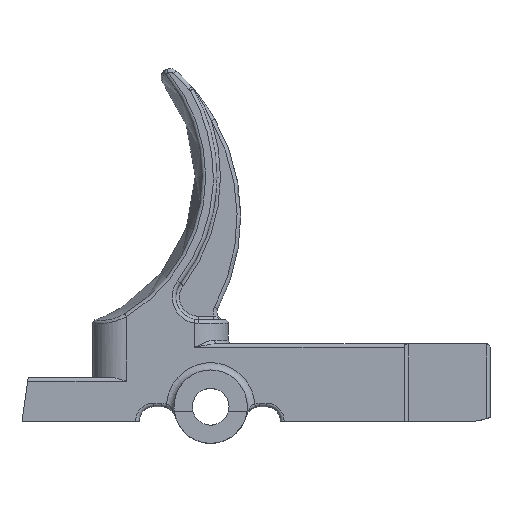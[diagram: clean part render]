
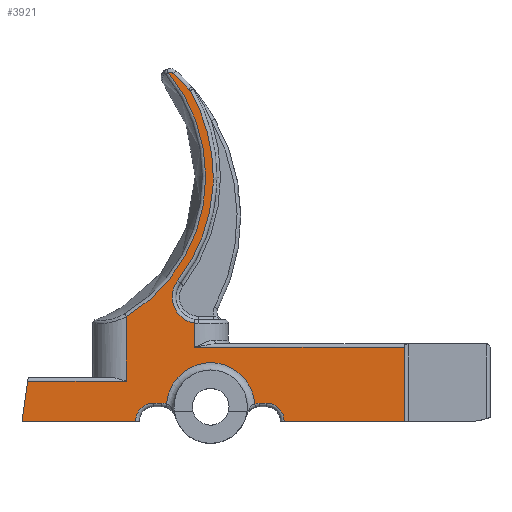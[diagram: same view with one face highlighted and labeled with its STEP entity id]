
A CAD part, top view. The second image highlights one B-rep face of the part: STEP entity #3921.
In plain terms, the highlighted planar face has unit normal (0, 0, 1).
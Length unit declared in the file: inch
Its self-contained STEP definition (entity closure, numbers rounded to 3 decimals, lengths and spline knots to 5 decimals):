
#43=DIRECTION('',(-1.,0.,0.));
#44=VECTOR('',#43,0.5164);
#45=CARTESIAN_POINT('',(1.19332,-0.3337,0.145));
#46=LINE('',#45,#44);
#96=CARTESIAN_POINT('',(0.59932,-0.332,0.145));
#97=DIRECTION('',(0.,0.,-1.));
#98=DIRECTION('',(0.,1.,0.));
#99=AXIS2_PLACEMENT_3D('',#96,#97,#98);
#104=CARTESIAN_POINT('',(0.57196,-0.332,0.145));
#105=DIRECTION('',(0.,0.,-1.));
#106=DIRECTION('',(-0.277,0.961,0.));
#107=AXIS2_PLACEMENT_3D('',#104,#105,#106);
#112=CARTESIAN_POINT('',(0.3617,-0.27001,0.145));
#113=DIRECTION('',(0.,0.,-1.));
#114=DIRECTION('',(-0.998,0.067,0.));
#115=AXIS2_PLACEMENT_3D('',#112,#113,#114);
#120=CARTESIAN_POINT('',(0.15144,-0.332,0.145));
#121=DIRECTION('',(0.,0.,-1.));
#122=DIRECTION('',(0.,1.,0.));
#123=AXIS2_PLACEMENT_3D('',#120,#121,#122);
#128=CARTESIAN_POINT('',(0.11722,-0.332,0.145));
#129=DIRECTION('',(0.,0.,-1.));
#130=DIRECTION('',(-1.,0.,0.));
#131=AXIS2_PLACEMENT_3D('',#128,#129,#130);
#136=DIRECTION('',(-0.139,-0.99,0.));
#137=VECTOR('',#136,0.17484);
#138=CARTESIAN_POINT('',(-0.42346,-0.16055,0.145));
#139=LINE('',#138,#137);
#143=CARTESIAN_POINT('',(-0.35887,0.71707,
0.145));
#144=DIRECTION('',(0.,0.,-1.));
#145=DIRECTION('',(0.769,0.639,0.));
#146=AXIS2_PLACEMENT_3D('',#143,#144,#145);
#151=CARTESIAN_POINT('',(0.18711,1.1428,0.145));
#152=DIRECTION('',(0.,0.,1.));
#153=DIRECTION('',(0.67,0.743,0.));
#154=AXIS2_PLACEMENT_3D('',#151,#152,#153);
#159=CARTESIAN_POINT('',(-0.35125,0.54559,0.145));
#160=DIRECTION('',(0.,0.,1.));
#161=DIRECTION('',(0.749,0.662,0.));
#162=AXIS2_PLACEMENT_3D('',#159,#160,#161);
#167=CARTESIAN_POINT('',(0.23327,1.06212,0.145));
#168=DIRECTION('',(0.,0.,1.));
#169=DIRECTION('',(0.864,0.503,0.));
#170=AXIS2_PLACEMENT_3D('',#167,#168,#169);
#175=CARTESIAN_POINT('',(-0.35887,0.71707,0.145));
#176=DIRECTION('',(0.,0.,1.));
#177=DIRECTION('',(1.,0.,0.));
#178=AXIS2_PLACEMENT_3D('',#175,#176,#177);
#183=CARTESIAN_POINT('',(-0.35887,0.71707,0.145));
#184=DIRECTION('',(0.,0.,1.));
#185=DIRECTION('',(0.998,-0.065,0.));
#186=AXIS2_PLACEMENT_3D('',#183,#184,#185);
#191=CARTESIAN_POINT('',(-0.35887,0.71707,0.145));
#192=DIRECTION('',(0.,0.,1.));
#193=DIRECTION('',(0.791,-0.611,0.));
#194=AXIS2_PLACEMENT_3D('',#191,#192,#193);
#199=CARTESIAN_POINT('',(0.30964,0.2005,0.145));
#200=DIRECTION('',(0.,0.,-1.));
#201=DIRECTION('',(-0.153,-0.988,0.));
#202=AXIS2_PLACEMENT_3D('',#199,#200,#201);
#231=DIRECTION('',(-1.,0.,0.));
#232=VECTOR('',#231,0.02736);
#233=CARTESIAN_POINT('',(0.59932,-0.2544,0.145));
#234=LINE('',#233,#232);
#692=DIRECTION('',(-1.,0.,0.));
#693=VECTOR('',#692,0.4874);
#694=CARTESIAN_POINT('',(0.03962,-0.3337,0.145));
#695=LINE('',#694,#693);
#1276=DIRECTION('',(0.,-1.,0.));
#1277=VECTOR('',#1276,0.3181);
#1278=CARTESIAN_POINT('',(1.19332,-0.0156,0.145));
#1279=LINE('',#1278,#1277);
#1327=DIRECTION('',(1.,0.,0.));
#1328=VECTOR('',#1327,0.90093);
#1329=CARTESIAN_POINT('',(0.29239,-0.0156,0.145));
#1330=LINE('',#1329,#1328);
#1844=DIRECTION('',(0.,-1.,0.));
#1845=VECTOR('',#1844,0.10432);
#1846=CARTESIAN_POINT('',(0.29239,0.08872,0.145));
#1847=LINE('',#1846,#1845);
#2919=DIRECTION('',(0.,1.,0.));
#2920=VECTOR('',#2919,0.27733);
#2921=CARTESIAN_POINT('',(0.,-0.16055,0.145));
#2922=LINE('',#2921,#2920);
#2972=DIRECTION('',(1.,0.,0.));
#2973=VECTOR('',#2972,0.42346);
#2974=CARTESIAN_POINT('',(-0.42346,-0.16055,0.145));
#2975=LINE('',#2974,#2973);
#3252=DIRECTION('',(0.,-1.,0.));
#3253=VECTOR('',#3252,0.0017);
#3254=CARTESIAN_POINT('',(0.03962,-0.332,0.145));
#3255=LINE('',#3254,#3253);
#3290=DIRECTION('',(-1.,0.,0.));
#3291=VECTOR('',#3290,0.03422);
#3292=CARTESIAN_POINT('',(0.15144,-0.2544,0.145));
#3293=LINE('',#3292,#3291);
#3335=DIRECTION('',(0.,1.,0.));
#3336=VECTOR('',#3335,0.0017);
#3337=CARTESIAN_POINT('',(0.67692,-0.3337,0.145));
#3338=LINE('',#3337,#3336);
#3377=CARTESIAN_POINT('',(1.19332,-0.3337,0.145));
#3378=CARTESIAN_POINT('',(0.67692,-0.3337,0.145));
#3379=VERTEX_POINT('',#3377);
#3380=VERTEX_POINT('',#3378);
#3416=CARTESIAN_POINT('',(0.03962,-0.3337,0.145));
#3417=VERTEX_POINT('',#3416);
#3418=CARTESIAN_POINT('',(-0.44778,-0.3337,0.145));
#3419=VERTEX_POINT('',#3418);
#3432=CARTESIAN_POINT('',(0.59932,-0.2544,0.145));
#3433=CARTESIAN_POINT('',(0.67692,-0.332,0.145));
#3434=VERTEX_POINT('',#3432);
#3435=VERTEX_POINT('',#3433);
#3436=CARTESIAN_POINT('',(1.19332,-0.0156,0.145));
#3437=VERTEX_POINT('',#3436);
#3438=CARTESIAN_POINT('',(0.29239,-0.0156,0.145));
#3439=VERTEX_POINT('',#3438);
#3440=CARTESIAN_POINT('',(0.29239,0.08872,0.145));
#3441=VERTEX_POINT('',#3440);
#3442=CARTESIAN_POINT('',(0.22015,0.26965,0.145));
#3443=VERTEX_POINT('',#3442);
#3444=CARTESIAN_POINT('',(0.37132,0.66944,0.145));
#3445=VERTEX_POINT('',#3444);
#3446=CARTESIAN_POINT('',(0.37287,0.71707,0.145));
#3447=VERTEX_POINT('',#3446);
#3448=CARTESIAN_POINT('',(0.27337,1.08548,0.145));
#3449=VERTEX_POINT('',#3448);
#3450=CARTESIAN_POINT('',(0.26804,1.09285,0.145));
#3451=VERTEX_POINT('',#3450);
#3452=CARTESIAN_POINT('',(0.20211,1.15944,0.145));
#3453=VERTEX_POINT('',#3452);
#3454=CARTESIAN_POINT('',(0.17927,1.16379,0.145));
#3455=VERTEX_POINT('',#3454);
#3456=CARTESIAN_POINT('',(0.,0.11678,
0.145));
#3457=VERTEX_POINT('',#3456);
#3458=CARTESIAN_POINT('',(0.,-0.16055,0.145));
#3459=VERTEX_POINT('',#3458);
#3460=CARTESIAN_POINT('',(-0.42346,-0.16055,0.145));
#3461=VERTEX_POINT('',#3460);
#3462=CARTESIAN_POINT('',(0.03962,-0.332,0.145));
#3463=VERTEX_POINT('',#3462);
#3464=CARTESIAN_POINT('',(0.11722,-0.2544,0.145));
#3465=VERTEX_POINT('',#3464);
#3466=CARTESIAN_POINT('',(0.15144,-0.2544,0.145));
#3467=VERTEX_POINT('',#3466);
#3468=CARTESIAN_POINT('',(0.17291,-0.25743,0.145));
#3469=VERTEX_POINT('',#3468);
#3470=CARTESIAN_POINT('',(0.55049,-0.25743,0.145));
#3471=VERTEX_POINT('',#3470);
#3472=CARTESIAN_POINT('',(0.57196,-0.2544,0.145));
#3473=VERTEX_POINT('',#3472);
#3865=CARTESIAN_POINT('',(0.,0.5937,0.145));
#3866=DIRECTION('',(0.,0.,-1.));
#3867=DIRECTION('',(-1.,0.,0.));
#3868=AXIS2_PLACEMENT_3D('',#3865,#3866,#3867);
#3869=PLANE('',#3868);
#3871=ORIENTED_EDGE('',*,*,#3870,.F.);
#3873=ORIENTED_EDGE('',*,*,#3872,.T.);
#3875=ORIENTED_EDGE('',*,*,#3874,.F.);
#3877=ORIENTED_EDGE('',*,*,#3876,.F.);
#3879=ORIENTED_EDGE('',*,*,#3878,.F.);
#3881=ORIENTED_EDGE('',*,*,#3880,.T.);
#3883=ORIENTED_EDGE('',*,*,#3882,.F.);
#3885=ORIENTED_EDGE('',*,*,#3884,.T.);
#3887=ORIENTED_EDGE('',*,*,#3886,.T.);
#3889=ORIENTED_EDGE('',*,*,#3888,.F.);
#3891=ORIENTED_EDGE('',*,*,#3890,.T.);
#3893=ORIENTED_EDGE('',*,*,#3892,.T.);
#3895=ORIENTED_EDGE('',*,*,#3894,.F.);
#3897=ORIENTED_EDGE('',*,*,#3896,.F.);
#3899=ORIENTED_EDGE('',*,*,#3898,.F.);
#3901=ORIENTED_EDGE('',*,*,#3900,.F.);
#3903=ORIENTED_EDGE('',*,*,#3902,.F.);
#3905=ORIENTED_EDGE('',*,*,#3904,.F.);
#3907=ORIENTED_EDGE('',*,*,#3906,.F.);
#3909=ORIENTED_EDGE('',*,*,#3908,.F.);
#3911=ORIENTED_EDGE('',*,*,#3910,.T.);
#3913=ORIENTED_EDGE('',*,*,#3912,.T.);
#3915=ORIENTED_EDGE('',*,*,#3914,.T.);
#3916=ORIENTED_EDGE('',*,*,#3843,.T.);
#3918=ORIENTED_EDGE('',*,*,#3917,.T.);
#3919=EDGE_LOOP('',(#3871,#3873,#3875,#3877,#3879,#3881,#3883,#3885,#3887,#3889,
#3891,#3893,#3895,#3897,#3899,#3901,#3903,#3905,#3907,#3909,#3911,#3913,#3915,
#3916,#3918));
#3920=FACE_OUTER_BOUND('',#3919,.F.);
#100=CIRCLE('',#99,0.0776);
#108=CIRCLE('',#107,0.0776);
#116=CIRCLE('',#115,0.18921);
#124=CIRCLE('',#123,0.0776);
#132=CIRCLE('',#131,0.0776);
#147=CIRCLE('',#146,0.69939);
#155=CIRCLE('',#154,0.0224);
#163=CIRCLE('',#162,0.82645);
#171=CIRCLE('',#170,0.0464);
#179=CIRCLE('',#178,0.73174);
#187=CIRCLE('',#186,0.73174);
#195=CIRCLE('',#194,0.73174);
#203=CIRCLE('',#202,0.1131);
#3843=EDGE_CURVE('',#3379,#3380,#46,.T.);
#3870=EDGE_CURVE('',#3434,#3435,#100,.T.);
#3872=EDGE_CURVE('',#3434,#3473,#234,.T.);
#3874=EDGE_CURVE('',#3471,#3473,#108,.T.);
#3876=EDGE_CURVE('',#3469,#3471,#116,.T.);
#3878=EDGE_CURVE('',#3467,#3469,#124,.T.);
#3880=EDGE_CURVE('',#3467,#3465,#3293,.T.);
#3882=EDGE_CURVE('',#3463,#3465,#132,.T.);
#3884=EDGE_CURVE('',#3463,#3417,#3255,.T.);
#3886=EDGE_CURVE('',#3417,#3419,#695,.T.);
#3888=EDGE_CURVE('',#3461,#3419,#139,.T.);
#3890=EDGE_CURVE('',#3461,#3459,#2975,.T.);
#3892=EDGE_CURVE('',#3459,#3457,#2922,.T.);
#3894=EDGE_CURVE('',#3455,#3457,#147,.T.);
#3896=EDGE_CURVE('',#3453,#3455,#155,.T.);
#3898=EDGE_CURVE('',#3451,#3453,#163,.T.);
#3900=EDGE_CURVE('',#3449,#3451,#171,.T.);
#3902=EDGE_CURVE('',#3447,#3449,#179,.T.);
#3904=EDGE_CURVE('',#3445,#3447,#187,.T.);
#3906=EDGE_CURVE('',#3443,#3445,#195,.T.);
#3908=EDGE_CURVE('',#3441,#3443,#203,.T.);
#3910=EDGE_CURVE('',#3441,#3439,#1847,.T.);
#3912=EDGE_CURVE('',#3439,#3437,#1330,.T.);
#3914=EDGE_CURVE('',#3437,#3379,#1279,.T.);
#3917=EDGE_CURVE('',#3380,#3435,#3338,.T.);
#3921=ADVANCED_FACE('',(#3920),#3869,.F.);
